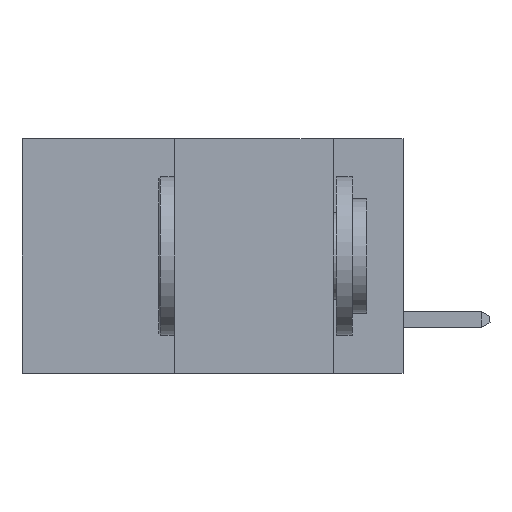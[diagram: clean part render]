
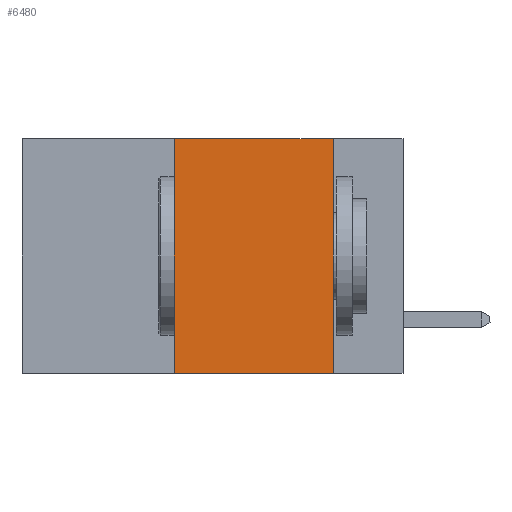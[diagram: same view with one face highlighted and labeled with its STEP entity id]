
A CAD part, left-side view. The second image highlights one B-rep face of the part: STEP entity #6480.
In plain terms, the highlighted planar face has unit normal (-1, 0, 0).
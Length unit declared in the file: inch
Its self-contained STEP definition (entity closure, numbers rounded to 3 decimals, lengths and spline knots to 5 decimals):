
#84 = VERTEX_POINT ( 'NONE', #14905 ) ;
#127 = CARTESIAN_POINT ( 'NONE',  ( 0., 0.6, 0. ) ) ;
#304 = DIRECTION ( 'NONE',  ( 1., 0., 0. ) ) ;
#945 = ORIENTED_EDGE ( 'NONE', *, *, #24605, .F. ) ;
#1020 = LINE ( 'NONE', #6476, #11298 ) ;
#1236 = CARTESIAN_POINT ( 'NONE',  ( 0., 0.6, -0.37 ) ) ;
#2073 = EDGE_CURVE ( 'NONE', #5240, #22730, #9374, .T. ) ;
#2244 = ORIENTED_EDGE ( 'NONE', *, *, #24243, .T. ) ;
#2713 = DIRECTION ( 'NONE',  ( 0., 0., 1. ) ) ;
#2754 = CARTESIAN_POINT ( 'NONE',  ( 0., 0.36, 0. ) ) ;
#2842 = CARTESIAN_POINT ( 'NONE',  ( 0., 0.36, 0. ) ) ;
#3353 = DIRECTION ( 'NONE',  ( 0., -1., 0. ) ) ;
#4371 = LINE ( 'NONE', #21926, #19531 ) ;
#5240 = VERTEX_POINT ( 'NONE', #25176 ) ;
#5921 = VECTOR ( 'NONE', #3353, 39.37008 ) ;
#6476 = CARTESIAN_POINT ( 'NONE',  ( 0., 0.6, 0. ) ) ;
#6480 = ADVANCED_FACE ( 'NONE', ( #15340 ), #22142, .F. ) ;
#8411 = DIRECTION ( 'NONE',  ( 0., 0., -1. ) ) ;
#9374 = LINE ( 'NONE', #2842, #24162 ) ;
#10649 = DIRECTION ( 'NONE',  ( 0., -1., 0. ) ) ;
#11298 = VECTOR ( 'NONE', #10649, 39.37008 ) ;
#14312 = EDGE_CURVE ( 'NONE', #21694, #84, #4371, .T. ) ;
#14541 = DIRECTION ( 'NONE',  ( 0., 0., -1. ) ) ;
#14905 = CARTESIAN_POINT ( 'NONE',  ( 0., 0.11, -0.37 ) ) ;
#15340 = FACE_OUTER_BOUND ( 'NONE', #21435, .T. ) ;
#15871 = LINE ( 'NONE', #1236, #5921 ) ;
#16993 = ORIENTED_EDGE ( 'NONE', *, *, #2073, .F. ) ;
#19531 = VECTOR ( 'NONE', #8411, 39.37008 ) ;
#20885 = ORIENTED_EDGE ( 'NONE', *, *, #14312, .F. ) ;
#21435 = EDGE_LOOP ( 'NONE', ( #20885, #945, #16993, #2244 ) ) ;
#21694 = VERTEX_POINT ( 'NONE', #22897 ) ;
#21926 = CARTESIAN_POINT ( 'NONE',  ( 0., 0.11, 0. ) ) ;
#22142 = PLANE ( 'NONE',  #24141 ) ;
#22730 = VERTEX_POINT ( 'NONE', #2754 ) ;
#22897 = CARTESIAN_POINT ( 'NONE',  ( 0., 0.11, 0. ) ) ;
#24141 = AXIS2_PLACEMENT_3D ( 'NONE', #127, #304, #14541 ) ;
#24162 = VECTOR ( 'NONE', #2713, 39.37008 ) ;
#24243 = EDGE_CURVE ( 'NONE', #5240, #84, #15871, .T. ) ;
#24605 = EDGE_CURVE ( 'NONE', #22730, #21694, #1020, .T. ) ;
#25176 = CARTESIAN_POINT ( 'NONE',  ( 0., 0.36, -0.37 ) ) ;
